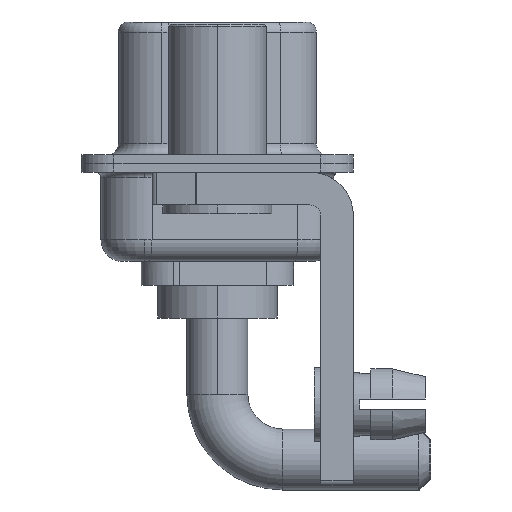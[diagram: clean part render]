
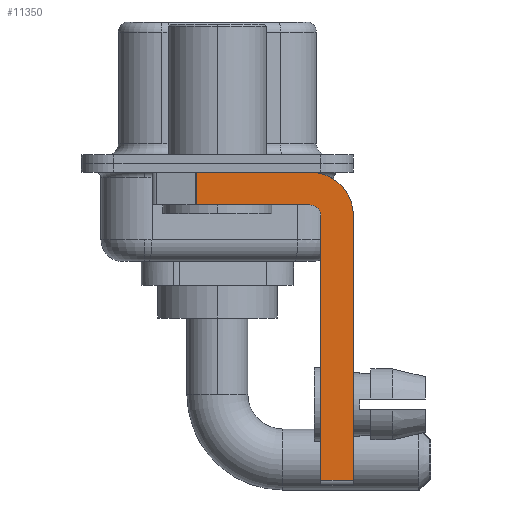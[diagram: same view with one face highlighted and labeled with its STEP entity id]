
A CAD part, left-side view. The second image highlights one B-rep face of the part: STEP entity #11350.
In plain terms, the highlighted planar face has unit normal (-1, 0, 0).
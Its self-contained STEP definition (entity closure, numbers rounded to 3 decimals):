
#42 = DIRECTION ( 'NONE',  ( 0., 0., -1. ) ) ;
#188 = PLANE ( 'NONE',  #7061 ) ;
#1093 = LINE ( 'NONE', #6812, #17768 ) ;
#1128 = CARTESIAN_POINT ( 'NONE',  ( -2.9, -4.75, -14.55 ) ) ;
#1360 = VECTOR ( 'NONE', #8464, 1000. ) ;
#1850 = VERTEX_POINT ( 'NONE', #16931 ) ;
#1918 = DIRECTION ( 'NONE',  ( 0., 0., -1. ) ) ;
#1951 = VERTEX_POINT ( 'NONE', #5714 ) ;
#1977 = VERTEX_POINT ( 'NONE', #1128 ) ;
#1999 = ORIENTED_EDGE ( 'NONE', *, *, #15965, .F. ) ;
#2142 = VECTOR ( 'NONE', #10392, 1000. ) ;
#2654 = DIRECTION ( 'NONE',  ( 0., 0., 1. ) ) ;
#2759 = CARTESIAN_POINT ( 'NONE',  ( -2.9, 3., -0.4 ) ) ;
#2875 = VECTOR ( 'NONE', #10673, 1000. ) ;
#3097 = DIRECTION ( 'NONE',  ( 1., 0., 0. ) ) ;
#3169 = AXIS2_PLACEMENT_3D ( 'NONE', #11636, #11927, #1918 ) ;
#5445 = CARTESIAN_POINT ( 'NONE',  ( -2.9, -4.25, -2.4 ) ) ;
#5543 = ORIENTED_EDGE ( 'NONE', *, *, #16525, .F. ) ;
#5714 = CARTESIAN_POINT ( 'NONE',  ( -2.9, -6.25, -2.4 ) ) ;
#5960 = CARTESIAN_POINT ( 'NONE',  ( -2.9, 0.978, -0.4 ) ) ;
#6112 = ORIENTED_EDGE ( 'NONE', *, *, #15661, .T. ) ;
#6348 = ORIENTED_EDGE ( 'NONE', *, *, #11467, .F. ) ;
#6812 = CARTESIAN_POINT ( 'NONE',  ( -2.9, -6.25, -2.4 ) ) ;
#7061 = AXIS2_PLACEMENT_3D ( 'NONE', #7218, #3097, #8521 ) ;
#7091 = VERTEX_POINT ( 'NONE', #14933 ) ;
#7218 = CARTESIAN_POINT ( 'NONE',  ( -2.9, -4.25, -2.4 ) ) ;
#7315 = LINE ( 'NONE', #15915, #2142 ) ;
#7574 = LINE ( 'NONE', #10376, #15062 ) ;
#7584 = LINE ( 'NONE', #9267, #2875 ) ;
#7982 = EDGE_LOOP ( 'NONE', ( #16295, #17499, #6348, #1999, #17474, #6112, #5543, #9649 ) ) ;
#8210 = EDGE_CURVE ( 'NONE', #13802, #12579, #7315, .T. ) ;
#8434 = FACE_OUTER_BOUND ( 'NONE', #7982, .T. ) ;
#8464 = DIRECTION ( 'NONE',  ( 0., -1., 0. ) ) ;
#8521 = DIRECTION ( 'NONE',  ( 0., 0., -1. ) ) ;
#8925 = EDGE_CURVE ( 'NONE', #13802, #7091, #11264, .T. ) ;
#9267 = CARTESIAN_POINT ( 'NONE',  ( -2.9, -4.25, -1.9 ) ) ;
#9464 = VERTEX_POINT ( 'NONE', #18276 ) ;
#9649 = ORIENTED_EDGE ( 'NONE', *, *, #12358, .F. ) ;
#9970 = DIRECTION ( 'NONE',  ( -1., 0., 0. ) ) ;
#10376 = CARTESIAN_POINT ( 'NONE',  ( -2.9, -4.25, -14.55 ) ) ;
#10392 = DIRECTION ( 'NONE',  ( 0., 0., -1. ) ) ;
#10673 = DIRECTION ( 'NONE',  ( 0., 1., 0. ) ) ;
#11264 = LINE ( 'NONE', #2759, #1360 ) ;
#11350 = ADVANCED_FACE ( 'NONE', ( #8434 ), #188, .F. ) ;
#11467 = EDGE_CURVE ( 'NONE', #9464, #12579, #7584, .T. ) ;
#11636 = CARTESIAN_POINT ( 'NONE',  ( -2.9, -4.25, -2.4 ) ) ;
#11927 = DIRECTION ( 'NONE',  ( 1., 0., 0. ) ) ;
#12358 = EDGE_CURVE ( 'NONE', #7091, #1951, #15714, .T. ) ;
#12579 = VERTEX_POINT ( 'NONE', #17741 ) ;
#13802 = VERTEX_POINT ( 'NONE', #5960 ) ;
#14159 = AXIS2_PLACEMENT_3D ( 'NONE', #5445, #9970, #18409 ) ;
#14903 = EDGE_CURVE ( 'NONE', #1977, #16336, #17052, .T. ) ;
#14933 = CARTESIAN_POINT ( 'NONE',  ( -2.9, -4.25, -0.4 ) ) ;
#15062 = VECTOR ( 'NONE', #16088, 1000. ) ;
#15076 = CIRCLE ( 'NONE', #14159, 0.5 ) ;
#15477 = CARTESIAN_POINT ( 'NONE',  ( -2.9, -4.75, -14.8 ) ) ;
#15661 = EDGE_CURVE ( 'NONE', #1977, #1850, #7574, .T. ) ;
#15714 = CIRCLE ( 'NONE', #3169, 2. ) ;
#15915 = CARTESIAN_POINT ( 'NONE',  ( -2.9, 0.978, -1.9 ) ) ;
#15965 = EDGE_CURVE ( 'NONE', #16336, #9464, #15076, .T. ) ;
#16088 = DIRECTION ( 'NONE',  ( 0., -1., 0. ) ) ;
#16295 = ORIENTED_EDGE ( 'NONE', *, *, #8925, .F. ) ;
#16336 = VERTEX_POINT ( 'NONE', #16543 ) ;
#16525 = EDGE_CURVE ( 'NONE', #1951, #1850, #1093, .T. ) ;
#16543 = CARTESIAN_POINT ( 'NONE',  ( -2.9, -4.75, -2.4 ) ) ;
#16931 = CARTESIAN_POINT ( 'NONE',  ( -2.9, -6.25, -14.55 ) ) ;
#17052 = LINE ( 'NONE', #15477, #17239 ) ;
#17239 = VECTOR ( 'NONE', #2654, 1000. ) ;
#17474 = ORIENTED_EDGE ( 'NONE', *, *, #14903, .F. ) ;
#17499 = ORIENTED_EDGE ( 'NONE', *, *, #8210, .T. ) ;
#17741 = CARTESIAN_POINT ( 'NONE',  ( -2.9, 0.978, -1.9 ) ) ;
#17768 = VECTOR ( 'NONE', #42, 1000. ) ;
#18276 = CARTESIAN_POINT ( 'NONE',  ( -2.9, -4.25, -1.9 ) ) ;
#18409 = DIRECTION ( 'NONE',  ( 0., 0., 1. ) ) ;
